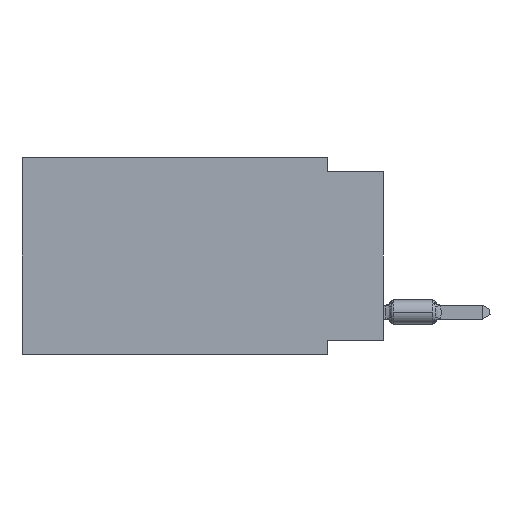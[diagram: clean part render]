
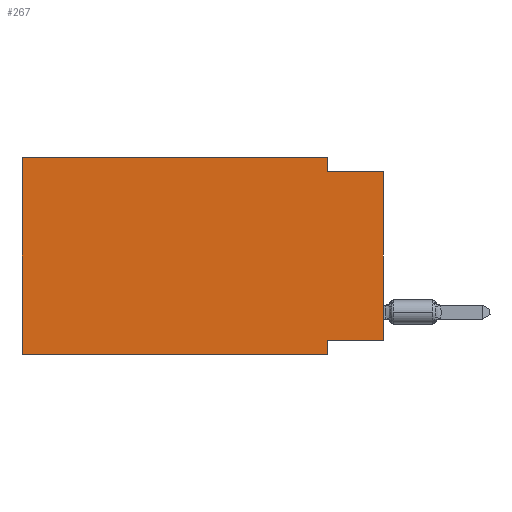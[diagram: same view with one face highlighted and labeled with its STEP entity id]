
A CAD part, left-side view. The second image highlights one B-rep face of the part: STEP entity #267.
In plain terms, the highlighted planar face has unit normal (-1, 0, 0).
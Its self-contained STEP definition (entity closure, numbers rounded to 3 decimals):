
#267 = ADVANCED_FACE ( 'NONE', ( #6013 ), #12876, .F. ) ;
#582 = DIRECTION ( 'NONE',  ( 0., 0., -1. ) ) ;
#776 = DIRECTION ( 'NONE',  ( 0., 1., 0. ) ) ;
#5110 = DIRECTION ( 'NONE',  ( 0., 0., 1. ) ) ;
#5336 = ORIENTED_EDGE ( 'NONE', *, *, #77481, .F. ) ;
#5835 = VERTEX_POINT ( 'NONE', #13895 ) ;
#5911 = LINE ( 'NONE', #64103, #16824 ) ;
#6013 = FACE_OUTER_BOUND ( 'NONE', #42541, .T. ) ;
#6615 = VERTEX_POINT ( 'NONE', #17445 ) ;
#9361 = EDGE_CURVE ( 'NONE', #54457, #23162, #55986, .T. ) ;
#10436 = EDGE_CURVE ( 'NONE', #55826, #5835, #48341, .T. ) ;
#11196 = CARTESIAN_POINT ( 'NONE',  ( 0., 16.383, 0. ) ) ;
#11706 = LINE ( 'NONE', #62242, #19103 ) ;
#11840 = AXIS2_PLACEMENT_3D ( 'NONE', #62223, #13278, #50092 ) ;
#12286 = CARTESIAN_POINT ( 'NONE',  ( 0., 0., -0.635 ) ) ;
#12660 = EDGE_CURVE ( 'NONE', #20449, #6615, #72667, .T. ) ;
#12766 = DIRECTION ( 'NONE',  ( 0., 0., 1. ) ) ;
#12876 = PLANE ( 'NONE',  #11840 ) ;
#13278 = DIRECTION ( 'NONE',  ( 1., 0., 0. ) ) ;
#13895 = CARTESIAN_POINT ( 'NONE',  ( 0., 2.54, -0.635 ) ) ;
#16824 = VECTOR ( 'NONE', #20444, 1000. ) ;
#17445 = CARTESIAN_POINT ( 'NONE',  ( 0., 16.383, 0. ) ) ;
#19103 = VECTOR ( 'NONE', #776, 1000. ) ;
#19581 = CARTESIAN_POINT ( 'NONE',  ( 0., 2.54, -8.89 ) ) ;
#19991 = CARTESIAN_POINT ( 'NONE',  ( 0., 0., -8.255 ) ) ;
#20444 = DIRECTION ( 'NONE',  ( 0., -1., 0. ) ) ;
#20449 = VERTEX_POINT ( 'NONE', #24534 ) ;
#23162 = VERTEX_POINT ( 'NONE', #52258 ) ;
#23584 = VECTOR ( 'NONE', #57947, 1000. ) ;
#24534 = CARTESIAN_POINT ( 'NONE',  ( 0., 16.383, -8.89 ) ) ;
#25706 = CARTESIAN_POINT ( 'NONE',  ( 0., 2.54, -8.255 ) ) ;
#26749 = DIRECTION ( 'NONE',  ( 0., -1., 0. ) ) ;
#30889 = ORIENTED_EDGE ( 'NONE', *, *, #10436, .F. ) ;
#32013 = ORIENTED_EDGE ( 'NONE', *, *, #12660, .F. ) ;
#38225 = CARTESIAN_POINT ( 'NONE',  ( 0., 0., 0. ) ) ;
#40163 = CARTESIAN_POINT ( 'NONE',  ( 0., 16.383, 0. ) ) ;
#42541 = EDGE_LOOP ( 'NONE', ( #76844, #5336, #30889, #64022, #32013, #47250, #59327, #51398 ) ) ;
#44405 = VECTOR ( 'NONE', #74183, 1000. ) ;
#45436 = VERTEX_POINT ( 'NONE', #19991 ) ;
#46234 = LINE ( 'NONE', #40163, #23584 ) ;
#47250 = ORIENTED_EDGE ( 'NONE', *, *, #71571, .T. ) ;
#48341 = LINE ( 'NONE', #79451, #44405 ) ;
#50092 = DIRECTION ( 'NONE',  ( 0., 0., -1. ) ) ;
#51398 = ORIENTED_EDGE ( 'NONE', *, *, #59803, .F. ) ;
#52258 = CARTESIAN_POINT ( 'NONE',  ( 0., 2.54, -8.89 ) ) ;
#52532 = VECTOR ( 'NONE', #26749, 1000. ) ;
#54457 = VERTEX_POINT ( 'NONE', #25706 ) ;
#55826 = VERTEX_POINT ( 'NONE', #78626 ) ;
#55986 = LINE ( 'NONE', #19581, #61087 ) ;
#57210 = EDGE_CURVE ( 'NONE', #45436, #62764, #68580, .T. ) ;
#57947 = DIRECTION ( 'NONE',  ( 0., -1., 0. ) ) ;
#59327 = ORIENTED_EDGE ( 'NONE', *, *, #9361, .F. ) ;
#59803 = EDGE_CURVE ( 'NONE', #45436, #54457, #11706, .T. ) ;
#61087 = VECTOR ( 'NONE', #582, 1000. ) ;
#62223 = CARTESIAN_POINT ( 'NONE',  ( 0., 16.383, 0. ) ) ;
#62242 = CARTESIAN_POINT ( 'NONE',  ( 0., 0., -8.255 ) ) ;
#62764 = VERTEX_POINT ( 'NONE', #12286 ) ;
#64022 = ORIENTED_EDGE ( 'NONE', *, *, #74761, .F. ) ;
#64103 = CARTESIAN_POINT ( 'NONE',  ( 0., 16.383, -8.89 ) ) ;
#67938 = VECTOR ( 'NONE', #12766, 1000. ) ;
#68580 = LINE ( 'NONE', #38225, #67938 ) ;
#70539 = VECTOR ( 'NONE', #5110, 1000. ) ;
#70807 = LINE ( 'NONE', #76853, #52532 ) ;
#71571 = EDGE_CURVE ( 'NONE', #20449, #23162, #5911, .T. ) ;
#72667 = LINE ( 'NONE', #11196, #70539 ) ;
#74183 = DIRECTION ( 'NONE',  ( 0., 0., -1. ) ) ;
#74761 = EDGE_CURVE ( 'NONE', #6615, #55826, #46234, .T. ) ;
#76844 = ORIENTED_EDGE ( 'NONE', *, *, #57210, .T. ) ;
#76853 = CARTESIAN_POINT ( 'NONE',  ( 0., 0., -0.635 ) ) ;
#77481 = EDGE_CURVE ( 'NONE', #5835, #62764, #70807, .T. ) ;
#78626 = CARTESIAN_POINT ( 'NONE',  ( 0., 2.54, 0. ) ) ;
#79451 = CARTESIAN_POINT ( 'NONE',  ( 0., 2.54, 0. ) ) ;
